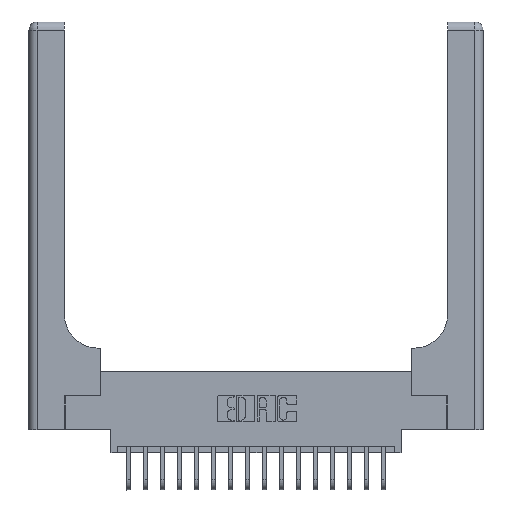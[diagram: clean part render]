
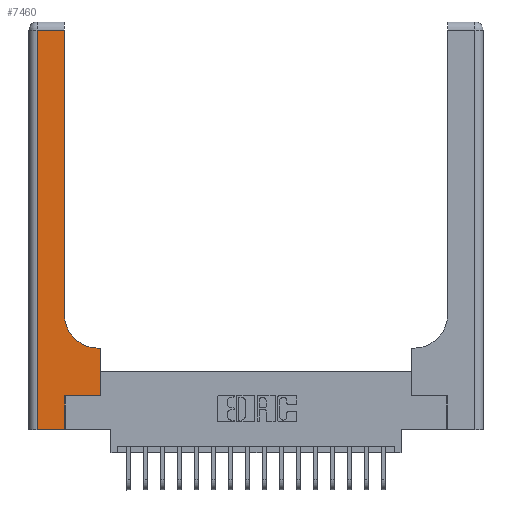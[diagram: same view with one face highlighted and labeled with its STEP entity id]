
A CAD part, top view. The second image highlights one B-rep face of the part: STEP entity #7460.
In plain terms, the highlighted planar face has unit normal (0, 0, 1).
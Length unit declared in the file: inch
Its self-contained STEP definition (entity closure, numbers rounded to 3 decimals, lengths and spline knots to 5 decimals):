
#15 = DIRECTION ( 'NONE',  ( -1., 0., 0. ) ) ;
#22 = EDGE_CURVE ( 'NONE', #11157, #14424, #8265, .T. ) ;
#204 = ORIENTED_EDGE ( 'NONE', *, *, #22, .T. ) ;
#428 = CARTESIAN_POINT ( 'NONE',  ( 0.265, 0., 0.37 ) ) ;
#560 = VECTOR ( 'NONE', #10132, 39.37008 ) ;
#769 = CARTESIAN_POINT ( 'NONE',  ( 0.26, 3., 0.37 ) ) ;
#1748 = CARTESIAN_POINT ( 'NONE',  ( 0., 0., 0.37 ) ) ;
#1814 = CARTESIAN_POINT ( 'NONE',  ( 0.51, 0.85, 0.37 ) ) ;
#1895 = DIRECTION ( 'NONE',  ( 0., -1., 0. ) ) ;
#1955 = VERTEX_POINT ( 'NONE', #2884 ) ;
#2884 = CARTESIAN_POINT ( 'NONE',  ( 0.51, 0.6, 0.37 ) ) ;
#3038 = CARTESIAN_POINT ( 'NONE',  ( 0.26, 2.94, 0.37 ) ) ;
#3292 = DIRECTION ( 'NONE',  ( 1., 0., 0. ) ) ;
#3404 = VERTEX_POINT ( 'NONE', #17701 ) ;
#3446 = PLANE ( 'NONE',  #3929 ) ;
#3637 = EDGE_CURVE ( 'NONE', #11341, #9021, #7925, .T. ) ;
#3929 = AXIS2_PLACEMENT_3D ( 'NONE', #7712, #13666, #4886 ) ;
#4260 = EDGE_LOOP ( 'NONE', ( #204, #15078, #13223, #6161, #15229, #10709, #9588, #12236, #16508 ) ) ;
#4886 = DIRECTION ( 'NONE',  ( -1., 0., 0. ) ) ;
#5359 = VERTEX_POINT ( 'NONE', #428 ) ;
#5544 = EDGE_CURVE ( 'NONE', #14424, #11341, #11334, .T. ) ;
#5682 = VECTOR ( 'NONE', #7813, 39.37008 ) ;
#5907 = EDGE_CURVE ( 'NONE', #9021, #5359, #10372, .T. ) ;
#6161 = ORIENTED_EDGE ( 'NONE', *, *, #5907, .T. ) ;
#6200 = CARTESIAN_POINT ( 'NONE',  ( 0.06, 3., 0.37 ) ) ;
#6381 = CARTESIAN_POINT ( 'NONE',  ( 0.528, 0.25, 0.37 ) ) ;
#7460 = ADVANCED_FACE ( 'NONE', ( #9174 ), #3446, .F. ) ;
#7712 = CARTESIAN_POINT ( 'NONE',  ( 0., 3., 0.37 ) ) ;
#7813 = DIRECTION ( 'NONE',  ( 0., 1., 0. ) ) ;
#7849 = VECTOR ( 'NONE', #8145, 39.37008 ) ;
#7925 = LINE ( 'NONE', #6200, #12348 ) ;
#7928 = DIRECTION ( 'NONE',  ( 0., 1., 0. ) ) ;
#8145 = DIRECTION ( 'NONE',  ( -1., 0., 0. ) ) ;
#8265 = LINE ( 'NONE', #769, #560 ) ;
#8279 = CARTESIAN_POINT ( 'NONE',  ( 0.265, 0.25, 0.37 ) ) ;
#8552 = CARTESIAN_POINT ( 'NONE',  ( 0.265, 0.25, 0.37 ) ) ;
#9021 = VERTEX_POINT ( 'NONE', #9953 ) ;
#9174 = FACE_OUTER_BOUND ( 'NONE', #4260, .T. ) ;
#9588 = ORIENTED_EDGE ( 'NONE', *, *, #11026, .T. ) ;
#9855 = VERTEX_POINT ( 'NONE', #10948 ) ;
#9953 = CARTESIAN_POINT ( 'NONE',  ( 0.06, 0., 0.37 ) ) ;
#10132 = DIRECTION ( 'NONE',  ( 0., 1., 0. ) ) ;
#10204 = CARTESIAN_POINT ( 'NONE',  ( 0.06, 2.94, 0.37 ) ) ;
#10372 = LINE ( 'NONE', #1748, #17242 ) ;
#10709 = ORIENTED_EDGE ( 'NONE', *, *, #15497, .T. ) ;
#10948 = CARTESIAN_POINT ( 'NONE',  ( 0.528, 0.6, 0.37 ) ) ;
#11026 = EDGE_CURVE ( 'NONE', #3404, #9855, #13952, .T. ) ;
#11157 = VERTEX_POINT ( 'NONE', #13954 ) ;
#11334 = LINE ( 'NONE', #12630, #7849 ) ;
#11341 = VERTEX_POINT ( 'NONE', #10204 ) ;
#11917 = LINE ( 'NONE', #8552, #15796 ) ;
#12015 = DIRECTION ( 'NONE',  ( 0., 0., -1. ) ) ;
#12236 = ORIENTED_EDGE ( 'NONE', *, *, #12721, .T. ) ;
#12348 = VECTOR ( 'NONE', #1895, 39.37008 ) ;
#12349 = CARTESIAN_POINT ( 'NONE',  ( 0.265, 0., 0.37 ) ) ;
#12630 = CARTESIAN_POINT ( 'NONE',  ( 0., 2.94, 0.37 ) ) ;
#12654 = VECTOR ( 'NONE', #7928, 39.37008 ) ;
#12721 = EDGE_CURVE ( 'NONE', #9855, #1955, #14117, .T. ) ;
#12813 = EDGE_CURVE ( 'NONE', #1955, #11157, #16574, .T. ) ;
#13223 = ORIENTED_EDGE ( 'NONE', *, *, #3637, .T. ) ;
#13666 = DIRECTION ( 'NONE',  ( 0., 0., -1. ) ) ;
#13952 = LINE ( 'NONE', #6381, #5682 ) ;
#13954 = CARTESIAN_POINT ( 'NONE',  ( 0.26, 0.85, 0.37 ) ) ;
#14117 = LINE ( 'NONE', #14702, #17910 ) ;
#14424 = VERTEX_POINT ( 'NONE', #3038 ) ;
#14702 = CARTESIAN_POINT ( 'NONE',  ( 0.26, 0.6, 0.37 ) ) ;
#15078 = ORIENTED_EDGE ( 'NONE', *, *, #5544, .T. ) ;
#15194 = EDGE_CURVE ( 'NONE', #5359, #16008, #16473, .T. ) ;
#15229 = ORIENTED_EDGE ( 'NONE', *, *, #15194, .T. ) ;
#15237 = AXIS2_PLACEMENT_3D ( 'NONE', #1814, #12015, #3292 ) ;
#15497 = EDGE_CURVE ( 'NONE', #16008, #3404, #11917, .T. ) ;
#15796 = VECTOR ( 'NONE', #18747, 39.37008 ) ;
#16008 = VERTEX_POINT ( 'NONE', #8279 ) ;
#16258 = DIRECTION ( 'NONE',  ( 1., 0., 0. ) ) ;
#16473 = LINE ( 'NONE', #12349, #12654 ) ;
#16508 = ORIENTED_EDGE ( 'NONE', *, *, #12813, .T. ) ;
#16574 = CIRCLE ( 'NONE', #15237, 0.25 ) ;
#17242 = VECTOR ( 'NONE', #16258, 39.37008 ) ;
#17701 = CARTESIAN_POINT ( 'NONE',  ( 0.528, 0.25, 0.37 ) ) ;
#17910 = VECTOR ( 'NONE', #15, 39.37008 ) ;
#18747 = DIRECTION ( 'NONE',  ( 1., 0., 0. ) ) ;
